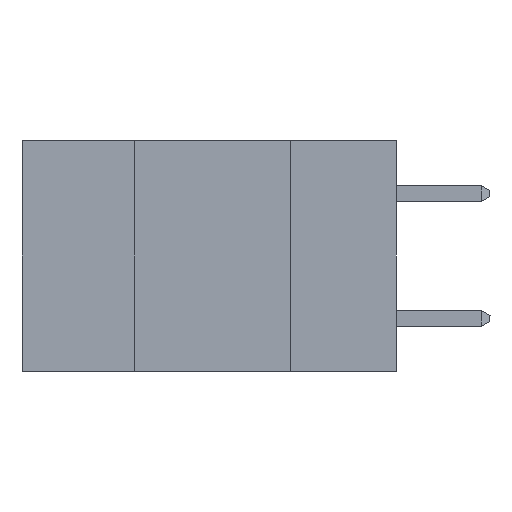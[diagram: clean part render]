
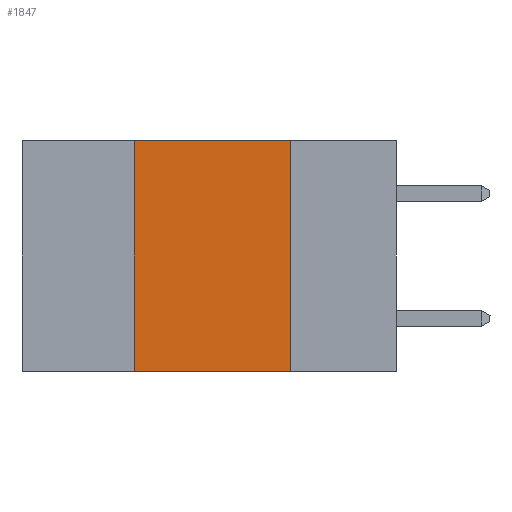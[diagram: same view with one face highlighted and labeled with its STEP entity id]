
A CAD part, left-side view. The second image highlights one B-rep face of the part: STEP entity #1847.
In plain terms, the highlighted planar face has unit normal (-1, 0, 0).
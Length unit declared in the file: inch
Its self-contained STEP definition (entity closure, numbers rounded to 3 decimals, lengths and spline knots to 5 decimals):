
#206 = EDGE_CURVE ( 'NONE', #1046, #9617, #2647, .T. ) ;
#275 = DIRECTION ( 'NONE',  ( 0., 0., 1. ) ) ;
#404 = PLANE ( 'NONE',  #2675 ) ;
#983 = EDGE_CURVE ( 'NONE', #9617, #2102, #1730, .T. ) ;
#1046 = VERTEX_POINT ( 'NONE', #6258 ) ;
#1182 = CARTESIAN_POINT ( 'NONE',  ( 0., 0.6, 0. ) ) ;
#1243 = CARTESIAN_POINT ( 'NONE',  ( 0., 0.6, -0.37 ) ) ;
#1730 = LINE ( 'NONE', #9568, #10123 ) ;
#1847 = ADVANCED_FACE ( 'NONE', ( #8105 ), #404, .F. ) ;
#1872 = DIRECTION ( 'NONE',  ( 1., 0., 0. ) ) ;
#2102 = VERTEX_POINT ( 'NONE', #7254 ) ;
#2321 = DIRECTION ( 'NONE',  ( 0., -1., 0. ) ) ;
#2647 = LINE ( 'NONE', #3920, #5620 ) ;
#2675 = AXIS2_PLACEMENT_3D ( 'NONE', #1182, #1872, #3911 ) ;
#3214 = VECTOR ( 'NONE', #3526, 39.37008 ) ;
#3291 = ORIENTED_EDGE ( 'NONE', *, *, #983, .F. ) ;
#3320 = ORIENTED_EDGE ( 'NONE', *, *, #206, .F. ) ;
#3332 = ORIENTED_EDGE ( 'NONE', *, *, #13504, .F. ) ;
#3437 = ORIENTED_EDGE ( 'NONE', *, *, #12810, .T. ) ;
#3509 = EDGE_LOOP ( 'NONE', ( #3291, #3320, #3332, #3437 ) ) ;
#3526 = DIRECTION ( 'NONE',  ( 0., -1., 0. ) ) ;
#3911 = DIRECTION ( 'NONE',  ( 0., 0., -1. ) ) ;
#3920 = CARTESIAN_POINT ( 'NONE',  ( 0., 0.6, 0. ) ) ;
#5620 = VECTOR ( 'NONE', #2321, 39.37008 ) ;
#5761 = CARTESIAN_POINT ( 'NONE',  ( 0., 0.17, 0. ) ) ;
#6170 = LINE ( 'NONE', #1243, #3214 ) ;
#6258 = CARTESIAN_POINT ( 'NONE',  ( 0., 0.42, 0. ) ) ;
#6735 = VERTEX_POINT ( 'NONE', #12288 ) ;
#7023 = CARTESIAN_POINT ( 'NONE',  ( 0., 0.42, -0.37 ) ) ;
#7254 = CARTESIAN_POINT ( 'NONE',  ( 0., 0.17, -0.37 ) ) ;
#8105 = FACE_OUTER_BOUND ( 'NONE', #3509, .T. ) ;
#9568 = CARTESIAN_POINT ( 'NONE',  ( 0., 0.17, -0.37 ) ) ;
#9617 = VERTEX_POINT ( 'NONE', #5761 ) ;
#10123 = VECTOR ( 'NONE', #11582, 39.37008 ) ;
#11268 = VECTOR ( 'NONE', #275, 39.37008 ) ;
#11582 = DIRECTION ( 'NONE',  ( 0., 0., -1. ) ) ;
#12288 = CARTESIAN_POINT ( 'NONE',  ( 0., 0.42, -0.37 ) ) ;
#12810 = EDGE_CURVE ( 'NONE', #6735, #2102, #6170, .T. ) ;
#13504 = EDGE_CURVE ( 'NONE', #6735, #1046, #13675, .T. ) ;
#13675 = LINE ( 'NONE', #7023, #11268 ) ;
